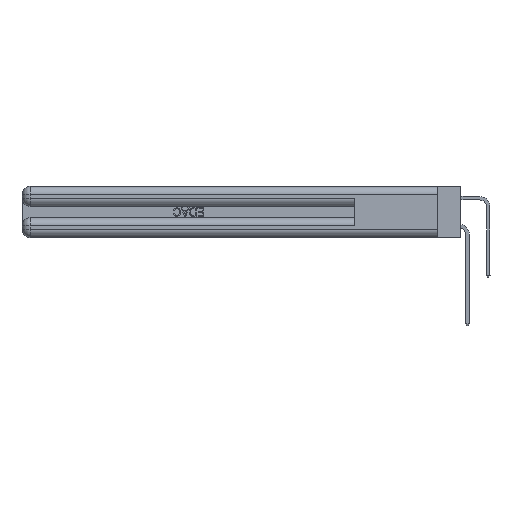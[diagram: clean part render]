
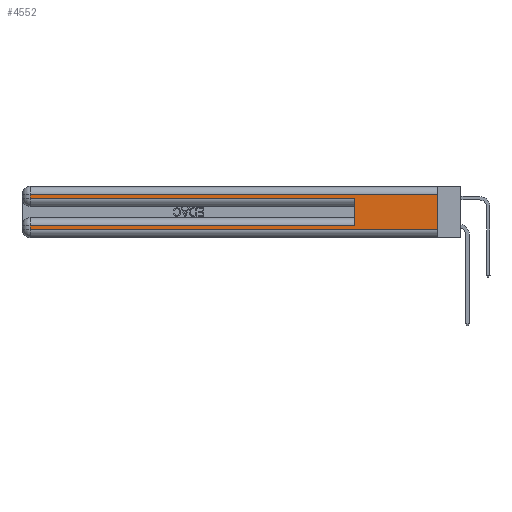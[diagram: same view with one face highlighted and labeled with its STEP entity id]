
A CAD part, left-side view. The second image highlights one B-rep face of the part: STEP entity #4552.
In plain terms, the highlighted planar face has unit normal (-1, 0, 0).
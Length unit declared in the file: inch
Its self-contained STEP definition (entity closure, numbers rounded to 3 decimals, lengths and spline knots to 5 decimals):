
#721 = VERTEX_POINT ( 'NONE', #14088 ) ;
#798 = EDGE_LOOP ( 'NONE', ( #31362, #4337, #27462, #37977, #17274, #25159, #39796, #35065 ) ) ;
#961 = CARTESIAN_POINT ( 'NONE',  ( 0., 2.94, 0.285 ) ) ;
#1075 = CARTESIAN_POINT ( 'NONE',  ( 0., 0., 0.085 ) ) ;
#1272 = VECTOR ( 'NONE', #29239, 39.37008 ) ;
#3363 = VERTEX_POINT ( 'NONE', #18119 ) ;
#3733 = VERTEX_POINT ( 'NONE', #19289 ) ;
#3819 = VECTOR ( 'NONE', #8596, 39.37008 ) ;
#4337 = ORIENTED_EDGE ( 'NONE', *, *, #10907, .T. ) ;
#4552 = ADVANCED_FACE ( 'NONE', ( #30076 ), #30906, .F. ) ;
#7244 = VECTOR ( 'NONE', #12575, 39.37008 ) ;
#8596 = DIRECTION ( 'NONE',  ( 0., 0., -1. ) ) ;
#8904 = DIRECTION ( 'NONE',  ( 0., 0., -1. ) ) ;
#10542 = CARTESIAN_POINT ( 'NONE',  ( 0., 0.6, 0.085 ) ) ;
#10907 = EDGE_CURVE ( 'NONE', #3363, #14029, #23053, .T. ) ;
#12360 = CARTESIAN_POINT ( 'NONE',  ( 0., 2.94, 0.37 ) ) ;
#12575 = DIRECTION ( 'NONE',  ( 0., 1., 0. ) ) ;
#12605 = LINE ( 'NONE', #27519, #3819 ) ;
#12619 = CARTESIAN_POINT ( 'NONE',  ( 0., 2.94, 0.06 ) ) ;
#13999 = DIRECTION ( 'NONE',  ( 0., -1., 0. ) ) ;
#14029 = VERTEX_POINT ( 'NONE', #44819 ) ;
#14088 = CARTESIAN_POINT ( 'NONE',  ( 0., 2.94, 0.085 ) ) ;
#14591 = VECTOR ( 'NONE', #23303, 39.37008 ) ;
#17071 = EDGE_CURVE ( 'NONE', #3363, #44870, #23597, .T. ) ;
#17274 = ORIENTED_EDGE ( 'NONE', *, *, #31723, .F. ) ;
#18119 = CARTESIAN_POINT ( 'NONE',  ( 0., 0., 0.31 ) ) ;
#19289 = CARTESIAN_POINT ( 'NONE',  ( 0., 0.6, 0.285 ) ) ;
#19563 = CARTESIAN_POINT ( 'NONE',  ( 0., 0., 0.37 ) ) ;
#19724 = DIRECTION ( 'NONE',  ( 1., 0., 0. ) ) ;
#20596 = EDGE_CURVE ( 'NONE', #14029, #29878, #12605, .T. ) ;
#22108 = CARTESIAN_POINT ( 'NONE',  ( 0., 0., 0.06 ) ) ;
#22800 = EDGE_CURVE ( 'NONE', #47360, #721, #39827, .T. ) ;
#23053 = LINE ( 'NONE', #46690, #7244 ) ;
#23303 = DIRECTION ( 'NONE',  ( 0., 0., 1. ) ) ;
#23597 = LINE ( 'NONE', #29495, #45156 ) ;
#25159 = ORIENTED_EDGE ( 'NONE', *, *, #22800, .T. ) ;
#25197 = AXIS2_PLACEMENT_3D ( 'NONE', #19563, #19724, #35136 ) ;
#25728 = VERTEX_POINT ( 'NONE', #12619 ) ;
#27462 = ORIENTED_EDGE ( 'NONE', *, *, #20596, .T. ) ;
#27519 = CARTESIAN_POINT ( 'NONE',  ( 0., 2.94, 0.37 ) ) ;
#29239 = DIRECTION ( 'NONE',  ( 0., -1., 0. ) ) ;
#29495 = CARTESIAN_POINT ( 'NONE',  ( 0., 0., 0.37 ) ) ;
#29813 = VECTOR ( 'NONE', #8904, 39.37008 ) ;
#29878 = VERTEX_POINT ( 'NONE', #961 ) ;
#29885 = VECTOR ( 'NONE', #30920, 39.37008 ) ;
#30076 = FACE_OUTER_BOUND ( 'NONE', #798, .T. ) ;
#30430 = CARTESIAN_POINT ( 'NONE',  ( 0., 0., 0.06 ) ) ;
#30538 = LINE ( 'NONE', #36457, #47578 ) ;
#30750 = CARTESIAN_POINT ( 'NONE',  ( 0., 0.6, 0.145 ) ) ;
#30906 = PLANE ( 'NONE',  #25197 ) ;
#30920 = DIRECTION ( 'NONE',  ( 0., 1., 0. ) ) ;
#31362 = ORIENTED_EDGE ( 'NONE', *, *, #17071, .F. ) ;
#31723 = EDGE_CURVE ( 'NONE', #47360, #3733, #34369, .T. ) ;
#34369 = LINE ( 'NONE', #30750, #14591 ) ;
#34532 = EDGE_CURVE ( 'NONE', #721, #25728, #42086, .T. ) ;
#35065 = ORIENTED_EDGE ( 'NONE', *, *, #40834, .T. ) ;
#35136 = DIRECTION ( 'NONE',  ( 0., 0., -1. ) ) ;
#36457 = CARTESIAN_POINT ( 'NONE',  ( 0., 0., 0.285 ) ) ;
#37977 = ORIENTED_EDGE ( 'NONE', *, *, #45423, .T. ) ;
#39796 = ORIENTED_EDGE ( 'NONE', *, *, #34532, .T. ) ;
#39827 = LINE ( 'NONE', #1075, #29885 ) ;
#40140 = DIRECTION ( 'NONE',  ( 0., 0., -1. ) ) ;
#40834 = EDGE_CURVE ( 'NONE', #25728, #44870, #47432, .T. ) ;
#42086 = LINE ( 'NONE', #12360, #29813 ) ;
#44819 = CARTESIAN_POINT ( 'NONE',  ( 0., 2.94, 0.31 ) ) ;
#44870 = VERTEX_POINT ( 'NONE', #30430 ) ;
#45156 = VECTOR ( 'NONE', #40140, 39.37008 ) ;
#45423 = EDGE_CURVE ( 'NONE', #29878, #3733, #30538, .T. ) ;
#46690 = CARTESIAN_POINT ( 'NONE',  ( 0., 0., 0.31 ) ) ;
#47360 = VERTEX_POINT ( 'NONE', #10542 ) ;
#47432 = LINE ( 'NONE', #22108, #1272 ) ;
#47578 = VECTOR ( 'NONE', #13999, 39.37008 ) ;
